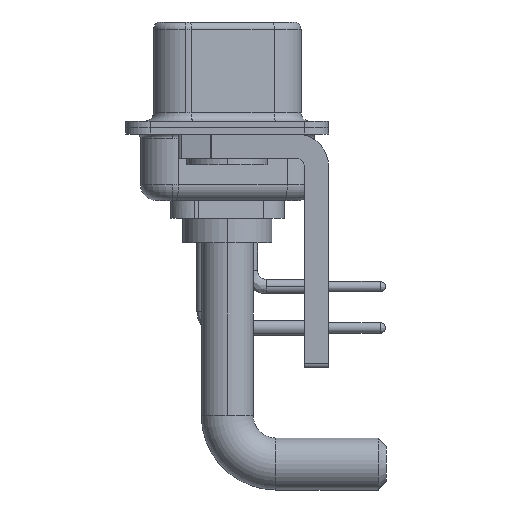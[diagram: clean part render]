
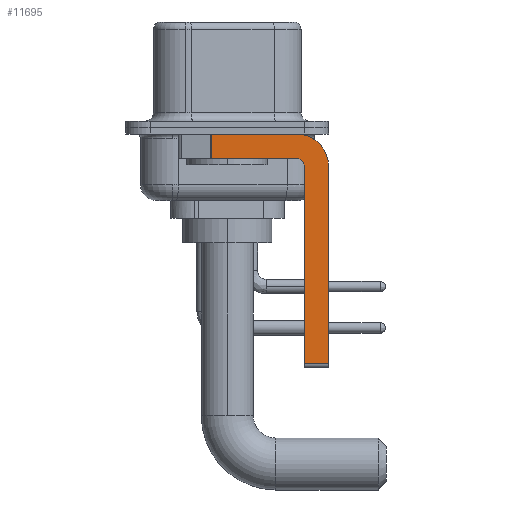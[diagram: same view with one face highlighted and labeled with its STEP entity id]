
A CAD part, left-side view. The second image highlights one B-rep face of the part: STEP entity #11695.
In plain terms, the highlighted planar face has unit normal (-1, 0, 0).
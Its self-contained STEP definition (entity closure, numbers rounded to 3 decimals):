
#50 = DIRECTION ( 'NONE',  ( 0., -1., 0. ) ) ;
#93 = CIRCLE ( 'NONE', #22965, 0.5 ) ;
#386 = PLANE ( 'NONE',  #1589 ) ;
#1053 = ORIENTED_EDGE ( 'NONE', *, *, #12752, .F. ) ;
#1099 = DIRECTION ( 'NONE',  ( 0., -1., 0. ) ) ;
#1399 = DIRECTION ( 'NONE',  ( 0., 0., -1. ) ) ;
#1589 = AXIS2_PLACEMENT_3D ( 'NONE', #14891, #5778, #22069 ) ;
#1692 = VERTEX_POINT ( 'NONE', #11882 ) ;
#1924 = VECTOR ( 'NONE', #9544, 1000. ) ;
#2072 = LINE ( 'NONE', #2291, #5088 ) ;
#2291 = CARTESIAN_POINT ( 'NONE',  ( -2.9, -4.25, -1.9 ) ) ;
#2413 = CARTESIAN_POINT ( 'NONE',  ( -2.9, -6.25, -14.55 ) ) ;
#2837 = ORIENTED_EDGE ( 'NONE', *, *, #4519, .T. ) ;
#2952 = EDGE_CURVE ( 'NONE', #13493, #8171, #5844, .T. ) ;
#3871 = VERTEX_POINT ( 'NONE', #11948 ) ;
#4092 = CARTESIAN_POINT ( 'NONE',  ( -2.9, -6.25, -2.4 ) ) ;
#4195 = CARTESIAN_POINT ( 'NONE',  ( -2.9, -4.25, -2.4 ) ) ;
#4378 = VERTEX_POINT ( 'NONE', #22751 ) ;
#4519 = EDGE_CURVE ( 'NONE', #1692, #13333, #21322, .T. ) ;
#5088 = VECTOR ( 'NONE', #18139, 1000. ) ;
#5196 = CARTESIAN_POINT ( 'NONE',  ( -2.9, 3., -0.4 ) ) ;
#5778 = DIRECTION ( 'NONE',  ( 1., 0., 0. ) ) ;
#5844 = LINE ( 'NONE', #20377, #1924 ) ;
#5859 = CIRCLE ( 'NONE', #12954, 2. ) ;
#5953 = DIRECTION ( 'NONE',  ( 0., 0., 1. ) ) ;
#6237 = EDGE_CURVE ( 'NONE', #23037, #13493, #5859, .T. ) ;
#6485 = CARTESIAN_POINT ( 'NONE',  ( -2.9, -4.25, -14.55 ) ) ;
#8171 = VERTEX_POINT ( 'NONE', #2413 ) ;
#8759 = CARTESIAN_POINT ( 'NONE',  ( -2.9, 0.978, -1.9 ) ) ;
#8894 = CARTESIAN_POINT ( 'NONE',  ( -2.9, -4.75, -14.8 ) ) ;
#9268 = CARTESIAN_POINT ( 'NONE',  ( -2.9, -4.25, -0.4 ) ) ;
#9544 = DIRECTION ( 'NONE',  ( 0., 0., -1. ) ) ;
#9685 = ORIENTED_EDGE ( 'NONE', *, *, #6237, .F. ) ;
#10037 = VECTOR ( 'NONE', #1099, 1000. ) ;
#10193 = VECTOR ( 'NONE', #50, 1000. ) ;
#10281 = EDGE_CURVE ( 'NONE', #3871, #4378, #93, .T. ) ;
#10284 = DIRECTION ( 'NONE',  ( 1., 0., 0. ) ) ;
#10440 = LINE ( 'NONE', #5196, #10193 ) ;
#10732 = CARTESIAN_POINT ( 'NONE',  ( -2.9, -4.75, -14.55 ) ) ;
#11334 = DIRECTION ( 'NONE',  ( 0., 0., 1. ) ) ;
#11677 = ORIENTED_EDGE ( 'NONE', *, *, #20112, .T. ) ;
#11695 = ADVANCED_FACE ( 'NONE', ( #12799 ), #386, .F. ) ;
#11846 = VECTOR ( 'NONE', #11334, 1000. ) ;
#11882 = CARTESIAN_POINT ( 'NONE',  ( -2.9, 0.978, -0.4 ) ) ;
#11948 = CARTESIAN_POINT ( 'NONE',  ( -2.9, -4.75, -2.4 ) ) ;
#12068 = CARTESIAN_POINT ( 'NONE',  ( -2.9, -4.25, -2.4 ) ) ;
#12752 = EDGE_CURVE ( 'NONE', #1692, #23037, #10440, .T. ) ;
#12799 = FACE_OUTER_BOUND ( 'NONE', #14321, .T. ) ;
#12806 = ORIENTED_EDGE ( 'NONE', *, *, #15173, .F. ) ;
#12954 = AXIS2_PLACEMENT_3D ( 'NONE', #12068, #10284, #1399 ) ;
#12980 = DIRECTION ( 'NONE',  ( -1., 0., 0. ) ) ;
#13333 = VERTEX_POINT ( 'NONE', #8759 ) ;
#13493 = VERTEX_POINT ( 'NONE', #4092 ) ;
#14321 = EDGE_LOOP ( 'NONE', ( #1053, #2837, #12806, #15757, #22945, #11677, #15101, #9685 ) ) ;
#14891 = CARTESIAN_POINT ( 'NONE',  ( -2.9, -4.25, -2.4 ) ) ;
#15101 = ORIENTED_EDGE ( 'NONE', *, *, #2952, .F. ) ;
#15173 = EDGE_CURVE ( 'NONE', #4378, #13333, #2072, .T. ) ;
#15757 = ORIENTED_EDGE ( 'NONE', *, *, #10281, .F. ) ;
#16076 = EDGE_CURVE ( 'NONE', #21309, #3871, #18738, .T. ) ;
#16267 = CARTESIAN_POINT ( 'NONE',  ( -2.9, 0.978, -1.9 ) ) ;
#18139 = DIRECTION ( 'NONE',  ( 0., 1., 0. ) ) ;
#18738 = LINE ( 'NONE', #8894, #11846 ) ;
#20112 = EDGE_CURVE ( 'NONE', #21309, #8171, #20921, .T. ) ;
#20178 = VECTOR ( 'NONE', #23217, 1000. ) ;
#20377 = CARTESIAN_POINT ( 'NONE',  ( -2.9, -6.25, -2.4 ) ) ;
#20921 = LINE ( 'NONE', #6485, #10037 ) ;
#21309 = VERTEX_POINT ( 'NONE', #10732 ) ;
#21322 = LINE ( 'NONE', #16267, #20178 ) ;
#22069 = DIRECTION ( 'NONE',  ( 0., 0., -1. ) ) ;
#22751 = CARTESIAN_POINT ( 'NONE',  ( -2.9, -4.25, -1.9 ) ) ;
#22945 = ORIENTED_EDGE ( 'NONE', *, *, #16076, .F. ) ;
#22965 = AXIS2_PLACEMENT_3D ( 'NONE', #4195, #12980, #5953 ) ;
#23037 = VERTEX_POINT ( 'NONE', #9268 ) ;
#23217 = DIRECTION ( 'NONE',  ( 0., 0., -1. ) ) ;
